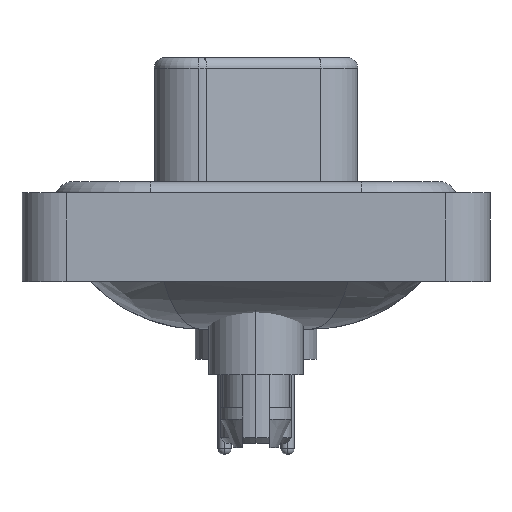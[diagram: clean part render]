
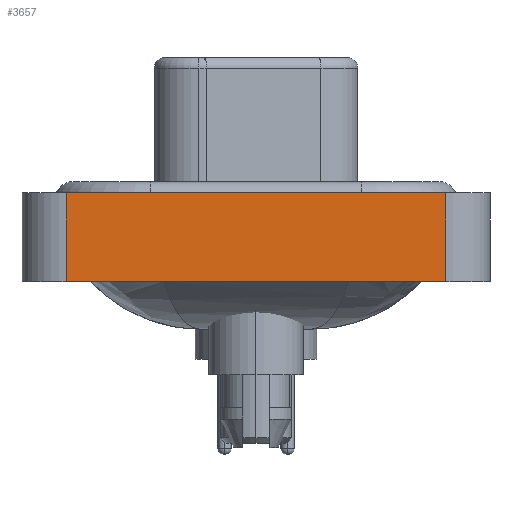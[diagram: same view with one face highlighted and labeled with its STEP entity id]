
A CAD part, left-side view. The second image highlights one B-rep face of the part: STEP entity #3657.
In plain terms, the highlighted planar face has unit normal (-1, 0, 0).
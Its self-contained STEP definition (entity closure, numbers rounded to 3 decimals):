
#514 = DIRECTION ( 'NONE',  ( 0., 0., 1. ) ) ;
#1525 = EDGE_CURVE ( 'NONE', #8360, #18152, #14534, .T. ) ;
#2468 = EDGE_CURVE ( 'NONE', #5626, #11560, #17161, .T. ) ;
#2786 = CARTESIAN_POINT ( 'NONE',  ( -7.35, -8.55, -3.6 ) ) ;
#2878 = LINE ( 'NONE', #15204, #16761 ) ;
#2997 = ORIENTED_EDGE ( 'NONE', *, *, #2468, .F. ) ;
#3038 = DIRECTION ( 'NONE',  ( -1., 0., 0. ) ) ;
#3657 = ADVANCED_FACE ( 'NONE', ( #22382 ), #8349, .T. ) ;
#4110 = EDGE_LOOP ( 'NONE', ( #11177, #22002, #2997, #17905 ) ) ;
#4817 = CARTESIAN_POINT ( 'NONE',  ( -7.35, -8.55, -3.6 ) ) ;
#4862 = DIRECTION ( 'NONE',  ( 0., -1., 0. ) ) ;
#5626 = VERTEX_POINT ( 'NONE', #6772 ) ;
#6772 = CARTESIAN_POINT ( 'NONE',  ( -7.35, 8.55, -3.6 ) ) ;
#7710 = VECTOR ( 'NONE', #15673, 1000. ) ;
#8349 = PLANE ( 'NONE',  #20481 ) ;
#8360 = VERTEX_POINT ( 'NONE', #2786 ) ;
#8914 = EDGE_CURVE ( 'NONE', #11560, #18152, #2878, .T. ) ;
#9711 = CARTESIAN_POINT ( 'NONE',  ( -7.35, 8.55, 0.4 ) ) ;
#9948 = CARTESIAN_POINT ( 'NONE',  ( -7.35, 8.55, -3.6 ) ) ;
#11177 = ORIENTED_EDGE ( 'NONE', *, *, #1525, .T. ) ;
#11488 = LINE ( 'NONE', #4817, #18344 ) ;
#11560 = VERTEX_POINT ( 'NONE', #9711 ) ;
#14534 = LINE ( 'NONE', #18199, #18612 ) ;
#15204 = CARTESIAN_POINT ( 'NONE',  ( -7.35, -8.55, 0.4 ) ) ;
#15673 = DIRECTION ( 'NONE',  ( 0., 0., 1. ) ) ;
#16761 = VECTOR ( 'NONE', #4862, 1000. ) ;
#17161 = LINE ( 'NONE', #9948, #7710 ) ;
#17905 = ORIENTED_EDGE ( 'NONE', *, *, #21372, .T. ) ;
#18134 = CARTESIAN_POINT ( 'NONE',  ( -7.35, -8.55, 0.4 ) ) ;
#18152 = VERTEX_POINT ( 'NONE', #18134 ) ;
#18199 = CARTESIAN_POINT ( 'NONE',  ( -7.35, -8.55, -3.6 ) ) ;
#18344 = VECTOR ( 'NONE', #22293, 1000. ) ;
#18612 = VECTOR ( 'NONE', #514, 1000. ) ;
#20481 = AXIS2_PLACEMENT_3D ( 'NONE', #20529, #3038, #22608 ) ;
#20529 = CARTESIAN_POINT ( 'NONE',  ( -7.35, -8.55, -3.6 ) ) ;
#21372 = EDGE_CURVE ( 'NONE', #5626, #8360, #11488, .T. ) ;
#22002 = ORIENTED_EDGE ( 'NONE', *, *, #8914, .F. ) ;
#22293 = DIRECTION ( 'NONE',  ( 0., -1., 0. ) ) ;
#22382 = FACE_OUTER_BOUND ( 'NONE', #4110, .T. ) ;
#22608 = DIRECTION ( 'NONE',  ( 0., 0., 1. ) ) ;
